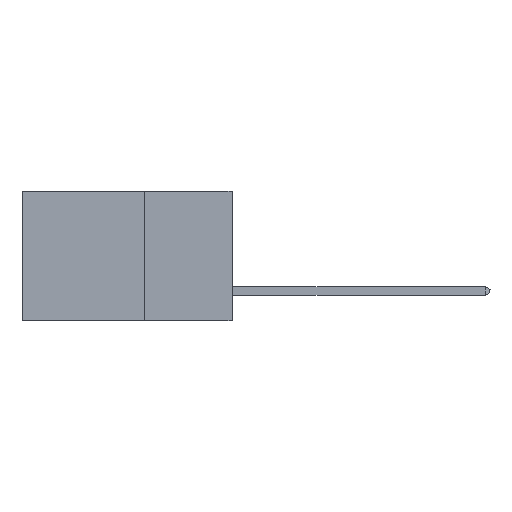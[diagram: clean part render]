
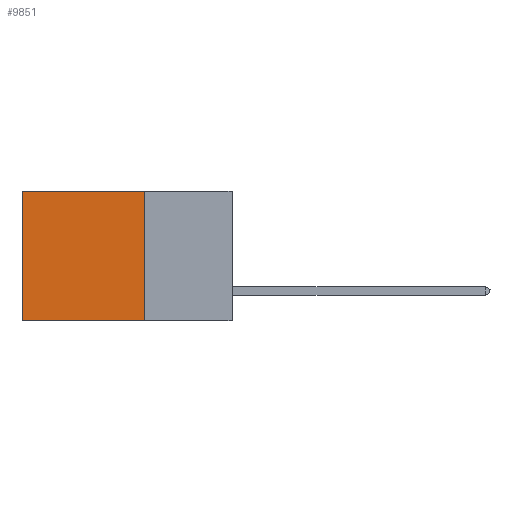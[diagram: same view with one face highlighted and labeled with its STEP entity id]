
A CAD part, left-side view. The second image highlights one B-rep face of the part: STEP entity #9851.
In plain terms, the highlighted planar face has unit normal (-1, 0, 0).
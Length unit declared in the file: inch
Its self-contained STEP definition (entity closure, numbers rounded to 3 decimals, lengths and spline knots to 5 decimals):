
#1897 = DIRECTION ( 'NONE',  ( 0., 0., -1. ) ) ;
#2911 = ORIENTED_EDGE ( 'NONE', *, *, #26452, .F. ) ;
#3678 = CARTESIAN_POINT ( 'NONE',  ( 0.2875, 0.6, -0.37 ) ) ;
#4510 = ORIENTED_EDGE ( 'NONE', *, *, #27886, .T. ) ;
#4957 = VECTOR ( 'NONE', #28434, 39.37008 ) ;
#9404 = LINE ( 'NONE', #10762, #27744 ) ;
#9768 = CARTESIAN_POINT ( 'NONE',  ( 0.2875, 0.25, 0. ) ) ;
#9851 = ADVANCED_FACE ( 'NONE', ( #16147 ), #14713, .F. ) ;
#10464 = VECTOR ( 'NONE', #28050, 39.37008 ) ;
#10762 = CARTESIAN_POINT ( 'NONE',  ( 0.2875, 0.25, 0. ) ) ;
#11523 = EDGE_CURVE ( 'NONE', #18138, #30130, #41989, .T. ) ;
#12106 = LINE ( 'NONE', #18732, #4957 ) ;
#13940 = EDGE_CURVE ( 'NONE', #26444, #18264, #39774, .T. ) ;
#14195 = AXIS2_PLACEMENT_3D ( 'NONE', #17992, #34425, #1897 ) ;
#14713 = PLANE ( 'NONE',  #14195 ) ;
#16147 = FACE_OUTER_BOUND ( 'NONE', #16558, .T. ) ;
#16548 = DIRECTION ( 'NONE',  ( 0., 0., -1. ) ) ;
#16558 = EDGE_LOOP ( 'NONE', ( #34319, #2911, #35159, #4510 ) ) ;
#17992 = CARTESIAN_POINT ( 'NONE',  ( 0.2875, 0.25, 0. ) ) ;
#18138 = VERTEX_POINT ( 'NONE', #18907 ) ;
#18264 = VERTEX_POINT ( 'NONE', #22289 ) ;
#18732 = CARTESIAN_POINT ( 'NONE',  ( 0.2875, 0.25, -0.37 ) ) ;
#18907 = CARTESIAN_POINT ( 'NONE',  ( 0.2875, 0.6, 0. ) ) ;
#22289 = CARTESIAN_POINT ( 'NONE',  ( 0.2875, 0.25, -0.37 ) ) ;
#26444 = VERTEX_POINT ( 'NONE', #9768 ) ;
#26452 = EDGE_CURVE ( 'NONE', #18264, #30130, #12106, .T. ) ;
#27744 = VECTOR ( 'NONE', #36882, 39.37008 ) ;
#27886 = EDGE_CURVE ( 'NONE', #26444, #18138, #9404, .T. ) ;
#28050 = DIRECTION ( 'NONE',  ( 0., 0., -1. ) ) ;
#28131 = VECTOR ( 'NONE', #16548, 39.37008 ) ;
#28434 = DIRECTION ( 'NONE',  ( 0., 1., 0. ) ) ;
#30130 = VERTEX_POINT ( 'NONE', #3678 ) ;
#31308 = CARTESIAN_POINT ( 'NONE',  ( 0.2875, 0.6, 0. ) ) ;
#34319 = ORIENTED_EDGE ( 'NONE', *, *, #11523, .T. ) ;
#34425 = DIRECTION ( 'NONE',  ( 1., 0., 0. ) ) ;
#35159 = ORIENTED_EDGE ( 'NONE', *, *, #13940, .F. ) ;
#36882 = DIRECTION ( 'NONE',  ( 0., 1., 0. ) ) ;
#38662 = CARTESIAN_POINT ( 'NONE',  ( 0.2875, 0.25, 0. ) ) ;
#39774 = LINE ( 'NONE', #38662, #28131 ) ;
#41989 = LINE ( 'NONE', #31308, #10464 ) ;
